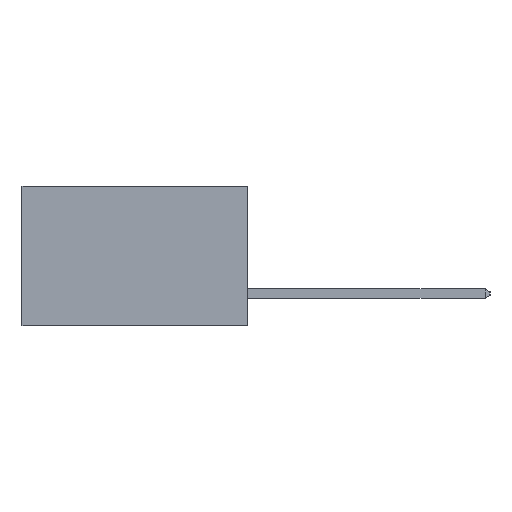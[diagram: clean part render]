
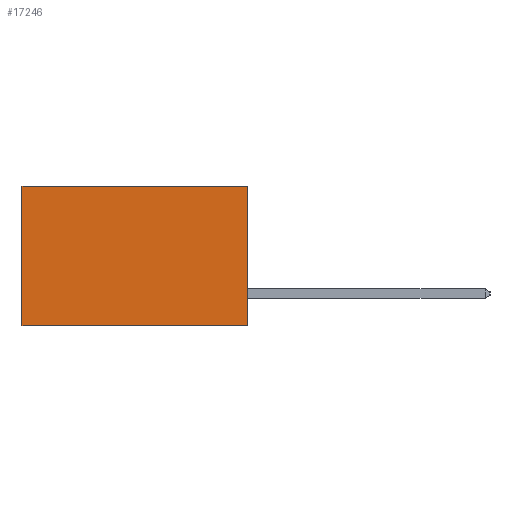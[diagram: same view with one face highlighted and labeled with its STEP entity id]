
A CAD part, left-side view. The second image highlights one B-rep face of the part: STEP entity #17246.
In plain terms, the highlighted planar face has unit normal (-1, 0, 0).
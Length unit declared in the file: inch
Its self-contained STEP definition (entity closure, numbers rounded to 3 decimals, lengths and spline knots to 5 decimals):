
#53 = EDGE_LOOP ( 'NONE', ( #9829, #18447, #16752, #12752 ) ) ;
#1027 = LINE ( 'NONE', #5740, #15418 ) ;
#4207 = VECTOR ( 'NONE', #4328, 39.37008 ) ;
#4328 = DIRECTION ( 'NONE',  ( 0., 0., -1. ) ) ;
#4720 = PLANE ( 'NONE',  #8791 ) ;
#4797 = LINE ( 'NONE', #13708, #4207 ) ;
#5740 = CARTESIAN_POINT ( 'NONE',  ( 0.2615, 0., 0. ) ) ;
#6111 = VERTEX_POINT ( 'NONE', #13819 ) ;
#6670 = DIRECTION ( 'NONE',  ( 0., 0., -1. ) ) ;
#7322 = LINE ( 'NONE', #23743, #21456 ) ;
#7996 = EDGE_CURVE ( 'NONE', #20678, #6111, #7322, .T. ) ;
#8791 = AXIS2_PLACEMENT_3D ( 'NONE', #21347, #17758, #6670 ) ;
#9072 = CARTESIAN_POINT ( 'NONE',  ( 0.2615, 0., -0.37 ) ) ;
#9829 = ORIENTED_EDGE ( 'NONE', *, *, #22945, .T. ) ;
#11260 = CARTESIAN_POINT ( 'NONE',  ( 0.2615, 0., -0.37 ) ) ;
#11297 = VERTEX_POINT ( 'NONE', #12592 ) ;
#11412 = DIRECTION ( 'NONE',  ( 0., 0., -1. ) ) ;
#11684 = VERTEX_POINT ( 'NONE', #23881 ) ;
#12592 = CARTESIAN_POINT ( 'NONE',  ( 0.2615, 0.6, 0. ) ) ;
#12752 = ORIENTED_EDGE ( 'NONE', *, *, #21678, .T. ) ;
#13487 = EDGE_CURVE ( 'NONE', #11684, #20678, #14487, .T. ) ;
#13708 = CARTESIAN_POINT ( 'NONE',  ( 0.2615, 0.6, -0.37 ) ) ;
#13819 = CARTESIAN_POINT ( 'NONE',  ( 0.2615, 0.6, -0.37 ) ) ;
#14487 = LINE ( 'NONE', #11260, #17959 ) ;
#15418 = VECTOR ( 'NONE', #16879, 39.37008 ) ;
#16752 = ORIENTED_EDGE ( 'NONE', *, *, #13487, .F. ) ;
#16879 = DIRECTION ( 'NONE',  ( 0., 1., 0. ) ) ;
#17246 = ADVANCED_FACE ( 'NONE', ( #23353 ), #4720, .F. ) ;
#17758 = DIRECTION ( 'NONE',  ( 1., 0., 0. ) ) ;
#17959 = VECTOR ( 'NONE', #11412, 39.37008 ) ;
#18447 = ORIENTED_EDGE ( 'NONE', *, *, #7996, .F. ) ;
#20678 = VERTEX_POINT ( 'NONE', #9072 ) ;
#21347 = CARTESIAN_POINT ( 'NONE',  ( 0.2615, 0., -0.37 ) ) ;
#21456 = VECTOR ( 'NONE', #23747, 39.37008 ) ;
#21678 = EDGE_CURVE ( 'NONE', #11684, #11297, #1027, .T. ) ;
#22945 = EDGE_CURVE ( 'NONE', #11297, #6111, #4797, .T. ) ;
#23353 = FACE_OUTER_BOUND ( 'NONE', #53, .T. ) ;
#23743 = CARTESIAN_POINT ( 'NONE',  ( 0.2615, 0., -0.37 ) ) ;
#23747 = DIRECTION ( 'NONE',  ( 0., 1., 0. ) ) ;
#23881 = CARTESIAN_POINT ( 'NONE',  ( 0.2615, 0., 0. ) ) ;
